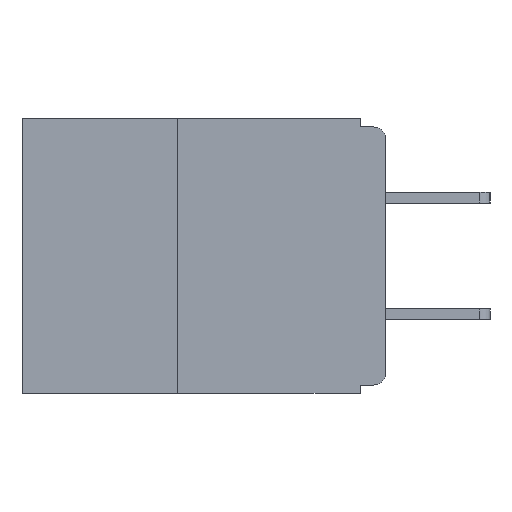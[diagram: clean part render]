
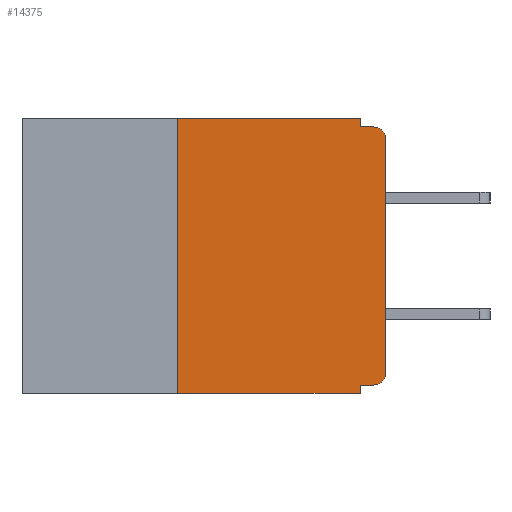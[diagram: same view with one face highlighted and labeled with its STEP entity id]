
A CAD part, left-side view. The second image highlights one B-rep face of the part: STEP entity #14375.
In plain terms, the highlighted planar face has unit normal (-1, 0, 0).
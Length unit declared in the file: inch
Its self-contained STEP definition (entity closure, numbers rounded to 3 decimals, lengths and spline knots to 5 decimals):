
#184 = LINE ( 'NONE', #3426, #20462 ) ;
#205 = CARTESIAN_POINT ( 'NONE',  ( 0., 0.031, -0.33 ) ) ;
#345 = VECTOR ( 'NONE', #7564, 39.37008 ) ;
#1400 = LINE ( 'NONE', #205, #18495 ) ;
#1660 = AXIS2_PLACEMENT_3D ( 'NONE', #26372, #11341, #28875 ) ;
#2784 = CARTESIAN_POINT ( 'NONE',  ( 0., 0., -0.305 ) ) ;
#3082 = CARTESIAN_POINT ( 'NONE',  ( 0., 0.25, -0.33 ) ) ;
#3351 = EDGE_LOOP ( 'NONE', ( #31992, #6519, #9048, #19629, #22204, #13086, #9426, #13463, #7697, #28154 ) ) ;
#3426 = CARTESIAN_POINT ( 'NONE',  ( 0., 0.25, -0.33 ) ) ;
#3657 = VERTEX_POINT ( 'NONE', #9636 ) ;
#4513 = EDGE_CURVE ( 'NONE', #13684, #22016, #19172, .T. ) ;
#4927 = EDGE_CURVE ( 'NONE', #8337, #27818, #14064, .T. ) ;
#5054 = VECTOR ( 'NONE', #31938, 39.37008 ) ;
#6519 = ORIENTED_EDGE ( 'NONE', *, *, #11763, .T. ) ;
#6935 = EDGE_CURVE ( 'NONE', #18263, #3657, #1400, .T. ) ;
#7184 = VERTEX_POINT ( 'NONE', #11279 ) ;
#7185 = EDGE_CURVE ( 'NONE', #22016, #12389, #23942, .T. ) ;
#7564 = DIRECTION ( 'NONE',  ( 0., 1., 0. ) ) ;
#7659 = CARTESIAN_POINT ( 'NONE',  ( 0., 0.031, -0.32 ) ) ;
#7697 = ORIENTED_EDGE ( 'NONE', *, *, #23418, .F. ) ;
#8337 = VERTEX_POINT ( 'NONE', #13343 ) ;
#8712 = CARTESIAN_POINT ( 'NONE',  ( 0., 0., 0. ) ) ;
#8831 = VERTEX_POINT ( 'NONE', #27723 ) ;
#9048 = ORIENTED_EDGE ( 'NONE', *, *, #4927, .F. ) ;
#9426 = ORIENTED_EDGE ( 'NONE', *, *, #27142, .T. ) ;
#9636 = CARTESIAN_POINT ( 'NONE',  ( 0., 0.031, -0.33 ) ) ;
#9657 = CARTESIAN_POINT ( 'NONE',  ( 0., 0.015, -0.32 ) ) ;
#9765 = CARTESIAN_POINT ( 'NONE',  ( 0., 0.437, 0. ) ) ;
#9824 = DIRECTION ( 'NONE',  ( 1., 0., 0. ) ) ;
#11279 = CARTESIAN_POINT ( 'NONE',  ( 0., 0.25, 0. ) ) ;
#11341 = DIRECTION ( 'NONE',  ( -1., 0., 0. ) ) ;
#11763 = EDGE_CURVE ( 'NONE', #12389, #27818, #18224, .T. ) ;
#12389 = VERTEX_POINT ( 'NONE', #29376 ) ;
#12450 = DIRECTION ( 'NONE',  ( 0., 0., -1. ) ) ;
#12713 = LINE ( 'NONE', #31738, #5054 ) ;
#13086 = ORIENTED_EDGE ( 'NONE', *, *, #29265, .F. ) ;
#13343 = CARTESIAN_POINT ( 'NONE',  ( 0., 0.031, -0.01 ) ) ;
#13463 = ORIENTED_EDGE ( 'NONE', *, *, #6935, .F. ) ;
#13684 = VERTEX_POINT ( 'NONE', #9657 ) ;
#13866 = DIRECTION ( 'NONE',  ( 0., 0., 1. ) ) ;
#14064 = LINE ( 'NONE', #16616, #28133 ) ;
#14375 = ADVANCED_FACE ( 'NONE', ( #31239 ), #27307, .F. ) ;
#15715 = LINE ( 'NONE', #22420, #28217 ) ;
#16610 = DIRECTION ( 'NONE',  ( 0., -1., 0. ) ) ;
#16616 = CARTESIAN_POINT ( 'NONE',  ( 0., 0., -0.01 ) ) ;
#17324 = VECTOR ( 'NONE', #13866, 39.37008 ) ;
#18036 = DIRECTION ( 'NONE',  ( 0., 0., -1. ) ) ;
#18106 = VECTOR ( 'NONE', #24821, 39.37008 ) ;
#18224 = CIRCLE ( 'NONE', #1660, 0.015 ) ;
#18263 = VERTEX_POINT ( 'NONE', #7659 ) ;
#18495 = VECTOR ( 'NONE', #18036, 39.37008 ) ;
#19172 = CIRCLE ( 'NONE', #31564, 0.015 ) ;
#19629 = ORIENTED_EDGE ( 'NONE', *, *, #30226, .F. ) ;
#19826 = LINE ( 'NONE', #20137, #345 ) ;
#20137 = CARTESIAN_POINT ( 'NONE',  ( 0., 0., -0.32 ) ) ;
#20426 = AXIS2_PLACEMENT_3D ( 'NONE', #24888, #9824, #27414 ) ;
#20462 = VECTOR ( 'NONE', #28611, 39.37008 ) ;
#22016 = VERTEX_POINT ( 'NONE', #2784 ) ;
#22204 = ORIENTED_EDGE ( 'NONE', *, *, #32012, .F. ) ;
#22420 = CARTESIAN_POINT ( 'NONE',  ( 0., 0.031, 0. ) ) ;
#22614 = DIRECTION ( 'NONE',  ( 0., 0., -1. ) ) ;
#22654 = DIRECTION ( 'NONE',  ( -1., 0., 0. ) ) ;
#22683 = CARTESIAN_POINT ( 'NONE',  ( 0., 0.015, -0.305 ) ) ;
#23418 = EDGE_CURVE ( 'NONE', #13684, #18263, #19826, .T. ) ;
#23942 = LINE ( 'NONE', #8712, #17324 ) ;
#24724 = LINE ( 'NONE', #9765, #18106 ) ;
#24737 = VERTEX_POINT ( 'NONE', #3082 ) ;
#24821 = DIRECTION ( 'NONE',  ( 0., -1., 0. ) ) ;
#24888 = CARTESIAN_POINT ( 'NONE',  ( 0., 0.437, 0. ) ) ;
#26372 = CARTESIAN_POINT ( 'NONE',  ( 0., 0.015, -0.025 ) ) ;
#27142 = EDGE_CURVE ( 'NONE', #24737, #3657, #12713, .T. ) ;
#27307 = PLANE ( 'NONE',  #20426 ) ;
#27414 = DIRECTION ( 'NONE',  ( 0., 0., -1. ) ) ;
#27723 = CARTESIAN_POINT ( 'NONE',  ( 0., 0.031, 0. ) ) ;
#27818 = VERTEX_POINT ( 'NONE', #32005 ) ;
#28133 = VECTOR ( 'NONE', #16610, 39.37008 ) ;
#28154 = ORIENTED_EDGE ( 'NONE', *, *, #4513, .T. ) ;
#28217 = VECTOR ( 'NONE', #12450, 39.37008 ) ;
#28611 = DIRECTION ( 'NONE',  ( 0., 0., 1. ) ) ;
#28875 = DIRECTION ( 'NONE',  ( 0., 0., -1. ) ) ;
#29265 = EDGE_CURVE ( 'NONE', #24737, #7184, #184, .T. ) ;
#29376 = CARTESIAN_POINT ( 'NONE',  ( 0., 0., -0.025 ) ) ;
#30226 = EDGE_CURVE ( 'NONE', #8831, #8337, #15715, .T. ) ;
#31239 = FACE_OUTER_BOUND ( 'NONE', #3351, .T. ) ;
#31564 = AXIS2_PLACEMENT_3D ( 'NONE', #22683, #22654, #22614 ) ;
#31738 = CARTESIAN_POINT ( 'NONE',  ( 0., 0.437, -0.33 ) ) ;
#31938 = DIRECTION ( 'NONE',  ( 0., -1., 0. ) ) ;
#31992 = ORIENTED_EDGE ( 'NONE', *, *, #7185, .T. ) ;
#32005 = CARTESIAN_POINT ( 'NONE',  ( 0., 0.015, -0.01 ) ) ;
#32012 = EDGE_CURVE ( 'NONE', #7184, #8831, #24724, .T. ) ;
